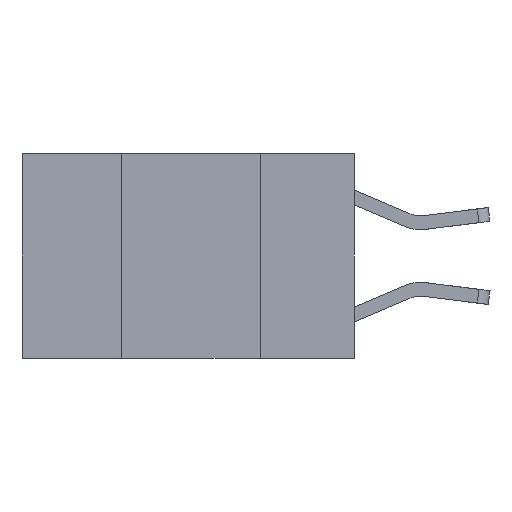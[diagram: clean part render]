
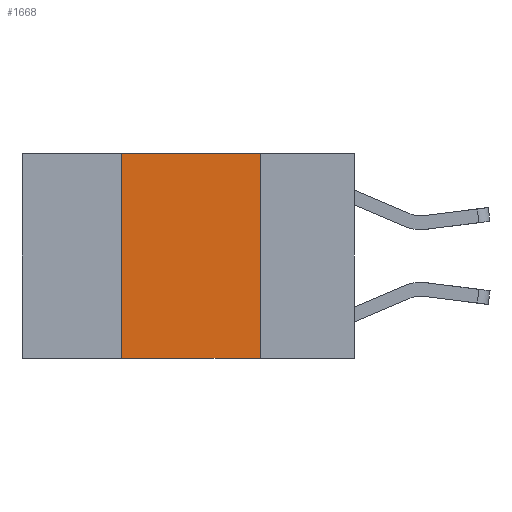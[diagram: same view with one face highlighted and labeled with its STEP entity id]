
A CAD part, left-side view. The second image highlights one B-rep face of the part: STEP entity #1668.
In plain terms, the highlighted planar face has unit normal (-1, 0, 0).
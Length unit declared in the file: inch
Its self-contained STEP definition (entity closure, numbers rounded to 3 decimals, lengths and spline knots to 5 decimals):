
#67 = LINE ( 'NONE', #2149, #8324 ) ;
#751 = EDGE_LOOP ( 'NONE', ( #7980, #5071, #2478, #9854 ) ) ;
#1144 = EDGE_CURVE ( 'NONE', #9767, #1251, #3727, .T. ) ;
#1241 = DIRECTION ( 'NONE',  ( 0., 0., -1. ) ) ;
#1251 = VERTEX_POINT ( 'NONE', #1389 ) ;
#1389 = CARTESIAN_POINT ( 'NONE',  ( 0., 0.17, -0.37 ) ) ;
#1668 = ADVANCED_FACE ( 'NONE', ( #4134 ), #2788, .F. ) ;
#2149 = CARTESIAN_POINT ( 'NONE',  ( 0., 0.6, 0. ) ) ;
#2478 = ORIENTED_EDGE ( 'NONE', *, *, #7346, .F. ) ;
#2774 = CARTESIAN_POINT ( 'NONE',  ( 0., 0.17, 0. ) ) ;
#2788 = PLANE ( 'NONE',  #9640 ) ;
#2960 = DIRECTION ( 'NONE',  ( 0., -1., 0. ) ) ;
#3435 = CARTESIAN_POINT ( 'NONE',  ( 0., 0.6, -0.37 ) ) ;
#3727 = LINE ( 'NONE', #7077, #9306 ) ;
#3983 = VECTOR ( 'NONE', #9259, 39.37008 ) ;
#4134 = FACE_OUTER_BOUND ( 'NONE', #751, .T. ) ;
#4338 = DIRECTION ( 'NONE',  ( 1., 0., 0. ) ) ;
#5071 = ORIENTED_EDGE ( 'NONE', *, *, #9554, .F. ) ;
#5085 = DIRECTION ( 'NONE',  ( 0., -1., 0. ) ) ;
#5366 = VECTOR ( 'NONE', #5085, 39.37008 ) ;
#5941 = DIRECTION ( 'NONE',  ( 0., 0., -1. ) ) ;
#6194 = CARTESIAN_POINT ( 'NONE',  ( 0., 0.42, -0.37 ) ) ;
#6236 = EDGE_CURVE ( 'NONE', #8843, #1251, #9545, .T. ) ;
#7077 = CARTESIAN_POINT ( 'NONE',  ( 0., 0.17, 0. ) ) ;
#7112 = VERTEX_POINT ( 'NONE', #8311 ) ;
#7346 = EDGE_CURVE ( 'NONE', #8843, #7112, #8222, .T. ) ;
#7980 = ORIENTED_EDGE ( 'NONE', *, *, #1144, .F. ) ;
#8098 = CARTESIAN_POINT ( 'NONE',  ( 0., 0.6, 0. ) ) ;
#8222 = LINE ( 'NONE', #8506, #3983 ) ;
#8311 = CARTESIAN_POINT ( 'NONE',  ( 0., 0.42, 0. ) ) ;
#8324 = VECTOR ( 'NONE', #2960, 39.37008 ) ;
#8506 = CARTESIAN_POINT ( 'NONE',  ( 0., 0.42, 0. ) ) ;
#8843 = VERTEX_POINT ( 'NONE', #6194 ) ;
#9259 = DIRECTION ( 'NONE',  ( 0., 0., 1. ) ) ;
#9306 = VECTOR ( 'NONE', #1241, 39.37008 ) ;
#9545 = LINE ( 'NONE', #3435, #5366 ) ;
#9554 = EDGE_CURVE ( 'NONE', #7112, #9767, #67, .T. ) ;
#9640 = AXIS2_PLACEMENT_3D ( 'NONE', #8098, #4338, #5941 ) ;
#9767 = VERTEX_POINT ( 'NONE', #2774 ) ;
#9854 = ORIENTED_EDGE ( 'NONE', *, *, #6236, .T. ) ;
